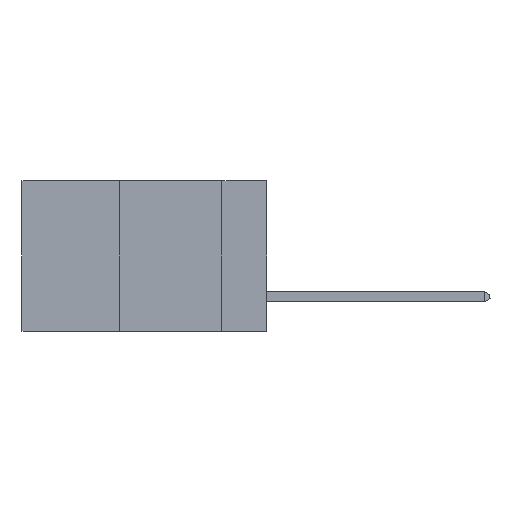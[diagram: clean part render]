
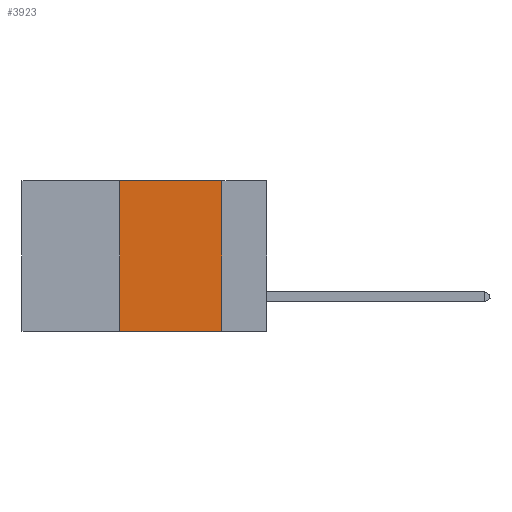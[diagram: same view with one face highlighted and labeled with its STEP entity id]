
A CAD part, left-side view. The second image highlights one B-rep face of the part: STEP entity #3923.
In plain terms, the highlighted planar face has unit normal (-1, 0, 0).
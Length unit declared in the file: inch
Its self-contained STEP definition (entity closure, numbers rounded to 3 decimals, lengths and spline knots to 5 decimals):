
#386 = VERTEX_POINT ( 'NONE', #6517 ) ;
#472 = ORIENTED_EDGE ( 'NONE', *, *, #7249, .T. ) ;
#596 = LINE ( 'NONE', #4992, #10206 ) ;
#708 = DIRECTION ( 'NONE',  ( 0., -1., 0. ) ) ;
#1869 = ORIENTED_EDGE ( 'NONE', *, *, #4953, .F. ) ;
#1916 = VERTEX_POINT ( 'NONE', #5850 ) ;
#2201 = VECTOR ( 'NONE', #6940, 39.37008 ) ;
#2228 = VECTOR ( 'NONE', #708, 39.37008 ) ;
#2425 = DIRECTION ( 'NONE',  ( 0., 0., 1. ) ) ;
#2481 = DIRECTION ( 'NONE',  ( 0., 0., -1. ) ) ;
#3273 = LINE ( 'NONE', #9893, #2228 ) ;
#3283 = CARTESIAN_POINT ( 'NONE',  ( 0., 0.11, -0.37 ) ) ;
#3636 = FACE_OUTER_BOUND ( 'NONE', #9933, .T. ) ;
#3923 = ADVANCED_FACE ( 'NONE', ( #3636 ), #6525, .F. ) ;
#4067 = CARTESIAN_POINT ( 'NONE',  ( 0., 0.6, 0. ) ) ;
#4368 = ORIENTED_EDGE ( 'NONE', *, *, #8931, .F. ) ;
#4953 = EDGE_CURVE ( 'NONE', #1916, #8065, #9882, .T. ) ;
#4992 = CARTESIAN_POINT ( 'NONE',  ( 0., 0.6, -0.37 ) ) ;
#5647 = EDGE_CURVE ( 'NONE', #386, #7563, #6451, .T. ) ;
#5850 = CARTESIAN_POINT ( 'NONE',  ( 0., 0.11, 0. ) ) ;
#6311 = CARTESIAN_POINT ( 'NONE',  ( 0., 0.36, 0. ) ) ;
#6451 = LINE ( 'NONE', #6311, #7641 ) ;
#6517 = CARTESIAN_POINT ( 'NONE',  ( 0., 0.36, -0.37 ) ) ;
#6525 = PLANE ( 'NONE',  #7635 ) ;
#6733 = CARTESIAN_POINT ( 'NONE',  ( 0., 0.11, 0. ) ) ;
#6940 = DIRECTION ( 'NONE',  ( 0., 0., -1. ) ) ;
#7249 = EDGE_CURVE ( 'NONE', #386, #8065, #596, .T. ) ;
#7263 = CARTESIAN_POINT ( 'NONE',  ( 0., 0.36, 0. ) ) ;
#7442 = DIRECTION ( 'NONE',  ( 1., 0., 0. ) ) ;
#7563 = VERTEX_POINT ( 'NONE', #7263 ) ;
#7635 = AXIS2_PLACEMENT_3D ( 'NONE', #4067, #7442, #2481 ) ;
#7641 = VECTOR ( 'NONE', #2425, 39.37008 ) ;
#8065 = VERTEX_POINT ( 'NONE', #3283 ) ;
#8173 = ORIENTED_EDGE ( 'NONE', *, *, #5647, .F. ) ;
#8931 = EDGE_CURVE ( 'NONE', #7563, #1916, #3273, .T. ) ;
#9244 = DIRECTION ( 'NONE',  ( 0., -1., 0. ) ) ;
#9882 = LINE ( 'NONE', #6733, #2201 ) ;
#9893 = CARTESIAN_POINT ( 'NONE',  ( 0., 0.6, 0. ) ) ;
#9933 = EDGE_LOOP ( 'NONE', ( #1869, #4368, #8173, #472 ) ) ;
#10206 = VECTOR ( 'NONE', #9244, 39.37008 ) ;
